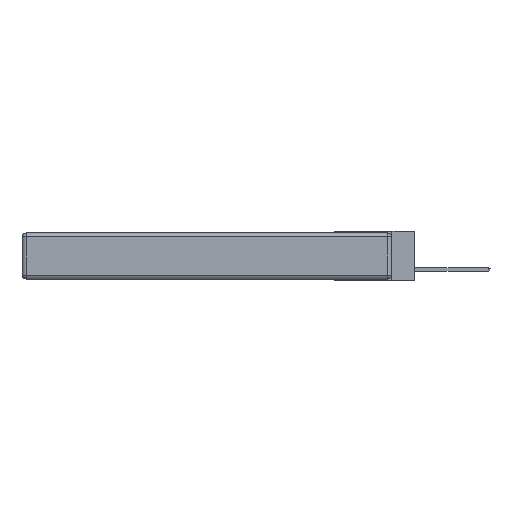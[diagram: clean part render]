
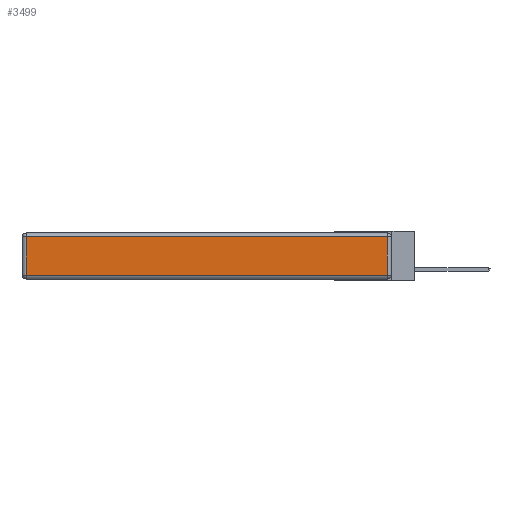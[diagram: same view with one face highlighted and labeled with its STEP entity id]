
A CAD part, left-side view. The second image highlights one B-rep face of the part: STEP entity #3499.
In plain terms, the highlighted planar face has unit normal (-1, 0, 0).
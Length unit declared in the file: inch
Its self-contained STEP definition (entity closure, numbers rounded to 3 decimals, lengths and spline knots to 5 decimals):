
#589 = VECTOR ( 'NONE', #19811, 39.37008 ) ;
#827 = EDGE_CURVE ( 'NONE', #15346, #8738, #8025, .T. ) ;
#1142 = VERTEX_POINT ( 'NONE', #6038 ) ;
#1169 = CARTESIAN_POINT ( 'NONE',  ( 0., 2.72, -0.343 ) ) ;
#1268 = DIRECTION ( 'NONE',  ( 0., 0., 1. ) ) ;
#1274 = ORIENTED_EDGE ( 'NONE', *, *, #14923, .T. ) ;
#2963 = CARTESIAN_POINT ( 'NONE',  ( 0., 2.72, -0.313 ) ) ;
#3151 = CARTESIAN_POINT ( 'NONE',  ( 0., 0., -0.313 ) ) ;
#3161 = CARTESIAN_POINT ( 'NONE',  ( 0., 2.75, -0.03 ) ) ;
#3499 = ADVANCED_FACE ( 'NONE', ( #16873 ), #4286, .T. ) ;
#4057 = ORIENTED_EDGE ( 'NONE', *, *, #827, .T. ) ;
#4286 = PLANE ( 'NONE',  #5178 ) ;
#4771 = DIRECTION ( 'NONE',  ( 0., -1., 0. ) ) ;
#5178 = AXIS2_PLACEMENT_3D ( 'NONE', #14804, #5775, #7228 ) ;
#5775 = DIRECTION ( 'NONE',  ( -1., 0., 0. ) ) ;
#5903 = CARTESIAN_POINT ( 'NONE',  ( 0., 0.03, -0.313 ) ) ;
#6038 = CARTESIAN_POINT ( 'NONE',  ( 0., 2.72, -0.03 ) ) ;
#7228 = DIRECTION ( 'NONE',  ( 0., 0., 1. ) ) ;
#8025 = LINE ( 'NONE', #3151, #13815 ) ;
#8738 = VERTEX_POINT ( 'NONE', #5903 ) ;
#12002 = DIRECTION ( 'NONE',  ( 0., 0., -1. ) ) ;
#12572 = VECTOR ( 'NONE', #12002, 39.37008 ) ;
#13815 = VECTOR ( 'NONE', #4771, 39.37008 ) ;
#14408 = VERTEX_POINT ( 'NONE', #16792 ) ;
#14804 = CARTESIAN_POINT ( 'NONE',  ( 0., 0., -0.343 ) ) ;
#14923 = EDGE_CURVE ( 'NONE', #14408, #1142, #17031, .T. ) ;
#15248 = CARTESIAN_POINT ( 'NONE',  ( 0., 0.03, -0.343 ) ) ;
#15346 = VERTEX_POINT ( 'NONE', #2963 ) ;
#16033 = VECTOR ( 'NONE', #1268, 39.37008 ) ;
#16034 = EDGE_CURVE ( 'NONE', #8738, #14408, #19919, .T. ) ;
#16720 = EDGE_LOOP ( 'NONE', ( #4057, #16798, #1274, #18134 ) ) ;
#16792 = CARTESIAN_POINT ( 'NONE',  ( 0., 0.03, -0.03 ) ) ;
#16798 = ORIENTED_EDGE ( 'NONE', *, *, #16034, .T. ) ;
#16873 = FACE_OUTER_BOUND ( 'NONE', #16720, .T. ) ;
#17031 = LINE ( 'NONE', #3161, #589 ) ;
#18134 = ORIENTED_EDGE ( 'NONE', *, *, #18250, .T. ) ;
#18250 = EDGE_CURVE ( 'NONE', #1142, #15346, #19301, .T. ) ;
#19301 = LINE ( 'NONE', #1169, #12572 ) ;
#19811 = DIRECTION ( 'NONE',  ( 0., 1., 0. ) ) ;
#19919 = LINE ( 'NONE', #15248, #16033 ) ;
